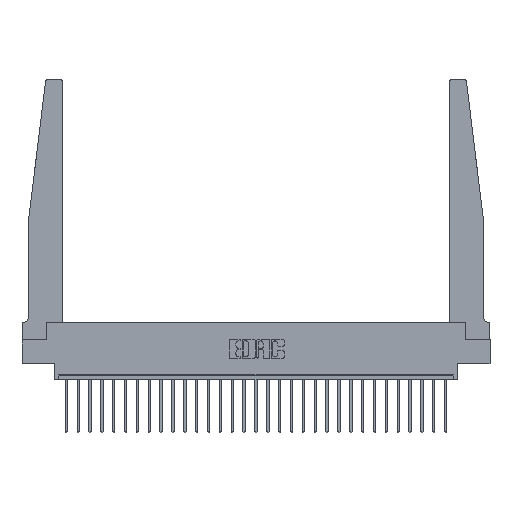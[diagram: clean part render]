
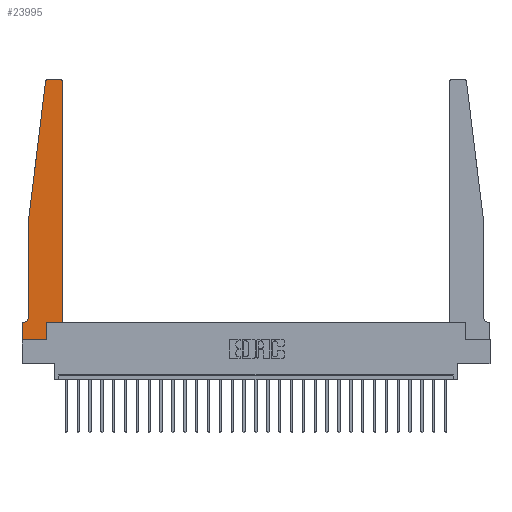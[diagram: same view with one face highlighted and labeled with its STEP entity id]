
A CAD part, top view. The second image highlights one B-rep face of the part: STEP entity #23995.
In plain terms, the highlighted planar face has unit normal (0, 0, 1).
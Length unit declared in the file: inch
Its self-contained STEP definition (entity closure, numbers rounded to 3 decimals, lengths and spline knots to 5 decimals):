
#101 = CARTESIAN_POINT ( 'NONE',  ( 0.015, 0.2375, 0.37 ) ) ;
#1660 = VECTOR ( 'NONE', #21999, 39.37008 ) ;
#1865 = LINE ( 'NONE', #8433, #6281 ) ;
#2936 = CARTESIAN_POINT ( 'NONE',  ( 0.065, 1.25, 0.37 ) ) ;
#2946 = LINE ( 'NONE', #7080, #1660 ) ;
#3023 = ORIENTED_EDGE ( 'NONE', *, *, #16589, .T. ) ;
#3166 = EDGE_CURVE ( 'NONE', #19661, #25735, #9652, .T. ) ;
#3373 = LINE ( 'NONE', #8254, #14221 ) ;
#3953 = EDGE_CURVE ( 'NONE', #21779, #18473, #4780, .T. ) ;
#4125 = CARTESIAN_POINT ( 'NONE',  ( 0., 0., 0.37 ) ) ;
#4203 = ORIENTED_EDGE ( 'NONE', *, *, #14254, .T. ) ;
#4204 = DIRECTION ( 'NONE',  ( -1., 0., 0. ) ) ;
#4245 = VECTOR ( 'NONE', #25683, 39.37008 ) ;
#4384 = VERTEX_POINT ( 'NONE', #24388 ) ;
#4780 = LINE ( 'NONE', #13141, #4907 ) ;
#4907 = VECTOR ( 'NONE', #21524, 39.37008 ) ;
#5101 = ORIENTED_EDGE ( 'NONE', *, *, #3953, .T. ) ;
#5239 = EDGE_CURVE ( 'NONE', #18473, #20666, #6199, .T. ) ;
#5373 = DIRECTION ( 'NONE',  ( 0., 0., 1. ) ) ;
#5426 = DIRECTION ( 'NONE',  ( 0., -1., 0. ) ) ;
#5432 = LINE ( 'NONE', #22148, #23500 ) ;
#5600 = VECTOR ( 'NONE', #7526, 39.37008 ) ;
#5661 = DIRECTION ( 'NONE',  ( 1., 0., 0. ) ) ;
#5679 = CARTESIAN_POINT ( 'NONE',  ( 0., 0., 0.37 ) ) ;
#6199 = LINE ( 'NONE', #4125, #15428 ) ;
#6280 = DIRECTION ( 'NONE',  ( 0., 0., -1. ) ) ;
#6281 = VECTOR ( 'NONE', #24971, 39.37008 ) ;
#6292 = DIRECTION ( 'NONE',  ( 1., 0., 0. ) ) ;
#7080 = CARTESIAN_POINT ( 'NONE',  ( 0.2605, 0.18, 0.37 ) ) ;
#7526 = DIRECTION ( 'NONE',  ( -1., 0., 0. ) ) ;
#7757 = VERTEX_POINT ( 'NONE', #9210 ) ;
#8254 = CARTESIAN_POINT ( 'NONE',  ( 0.065, 1.25, 0.37 ) ) ;
#8343 = CARTESIAN_POINT ( 'NONE',  ( 0.2605, 0.18, 0.37 ) ) ;
#8433 = CARTESIAN_POINT ( 'NONE',  ( 0.425, 0.18, 0.37 ) ) ;
#9161 = VECTOR ( 'NONE', #5661, 39.37008 ) ;
#9210 = CARTESIAN_POINT ( 'NONE',  ( 0.065, 0.2375, 0.37 ) ) ;
#9436 = AXIS2_PLACEMENT_3D ( 'NONE', #11283, #17607, #25920 ) ;
#9564 = LINE ( 'NONE', #26242, #5600 ) ;
#9652 = CIRCLE ( 'NONE', #13168, 0.03 ) ;
#10491 = CARTESIAN_POINT ( 'NONE',  ( 0.425, 2.72, 0.37 ) ) ;
#10650 = VERTEX_POINT ( 'NONE', #2936 ) ;
#10779 = DIRECTION ( 'NONE',  ( 0., 0., 1. ) ) ;
#10784 = EDGE_LOOP ( 'NONE', ( #18239, #18082, #24838, #4203, #22296, #5101, #16440, #13795, #3023, #15134, #13381, #20761 ) ) ;
#10858 = VERTEX_POINT ( 'NONE', #10491 ) ;
#10872 = EDGE_CURVE ( 'NONE', #7757, #21779, #24179, .T. ) ;
#10922 = PLANE ( 'NONE',  #18809 ) ;
#11168 = EDGE_CURVE ( 'NONE', #24058, #11967, #1865, .T. ) ;
#11248 = CARTESIAN_POINT ( 'NONE',  ( 0.27653, 2.75, 0.37 ) ) ;
#11283 = CARTESIAN_POINT ( 'NONE',  ( 0.395, 2.72, 0.37 ) ) ;
#11967 = VERTEX_POINT ( 'NONE', #13447 ) ;
#12859 = CARTESIAN_POINT ( 'NONE',  ( 0., 0.1875, 0.37 ) ) ;
#12895 = DIRECTION ( 'NONE',  ( 0., -1., 0. ) ) ;
#13141 = CARTESIAN_POINT ( 'NONE',  ( 0.065, 0.1875, 0.37 ) ) ;
#13168 = AXIS2_PLACEMENT_3D ( 'NONE', #20211, #5373, #19806 ) ;
#13298 = CARTESIAN_POINT ( 'NONE',  ( 0.395, 2.75, 0.37 ) ) ;
#13381 = ORIENTED_EDGE ( 'NONE', *, *, #21760, .T. ) ;
#13386 = LINE ( 'NONE', #19452, #4245 ) ;
#13447 = CARTESIAN_POINT ( 'NONE',  ( 0.425, 0.18, 0.37 ) ) ;
#13795 = ORIENTED_EDGE ( 'NONE', *, *, #13977, .T. ) ;
#13977 = EDGE_CURVE ( 'NONE', #20666, #4384, #16062, .T. ) ;
#14221 = VECTOR ( 'NONE', #5426, 39.37008 ) ;
#14254 = EDGE_CURVE ( 'NONE', #10650, #7757, #3373, .T. ) ;
#14568 = EDGE_CURVE ( 'NONE', #10858, #25699, #19537, .T. ) ;
#15134 = ORIENTED_EDGE ( 'NONE', *, *, #11168, .T. ) ;
#15428 = VECTOR ( 'NONE', #12895, 39.37008 ) ;
#15886 = AXIS2_PLACEMENT_3D ( 'NONE', #101, #6280, #4204 ) ;
#16062 = LINE ( 'NONE', #24386, #9161 ) ;
#16440 = ORIENTED_EDGE ( 'NONE', *, *, #5239, .T. ) ;
#16589 = EDGE_CURVE ( 'NONE', #4384, #24058, #2946, .T. ) ;
#17607 = DIRECTION ( 'NONE',  ( 0., 0., 1. ) ) ;
#18062 = DIRECTION ( 'NONE',  ( 0., 1., 0. ) ) ;
#18082 = ORIENTED_EDGE ( 'NONE', *, *, #3166, .T. ) ;
#18239 = ORIENTED_EDGE ( 'NONE', *, *, #22589, .T. ) ;
#18473 = VERTEX_POINT ( 'NONE', #27048 ) ;
#18809 = AXIS2_PLACEMENT_3D ( 'NONE', #12859, #10779, #6292 ) ;
#19452 = CARTESIAN_POINT ( 'NONE',  ( 0.065, 1.25, 0.37 ) ) ;
#19537 = CIRCLE ( 'NONE', #9436, 0.03 ) ;
#19661 = VERTEX_POINT ( 'NONE', #11248 ) ;
#19806 = DIRECTION ( 'NONE',  ( 1., 0., 0. ) ) ;
#20211 = CARTESIAN_POINT ( 'NONE',  ( 0.27653, 2.72, 0.37 ) ) ;
#20666 = VERTEX_POINT ( 'NONE', #5679 ) ;
#20761 = ORIENTED_EDGE ( 'NONE', *, *, #14568, .T. ) ;
#21524 = DIRECTION ( 'NONE',  ( -1., 0., 0. ) ) ;
#21607 = EDGE_CURVE ( 'NONE', #25735, #10650, #13386, .T. ) ;
#21760 = EDGE_CURVE ( 'NONE', #11967, #10858, #5432, .T. ) ;
#21779 = VERTEX_POINT ( 'NONE', #22276 ) ;
#21933 = CARTESIAN_POINT ( 'NONE',  ( 0.24675, 2.72367, 0.37 ) ) ;
#21999 = DIRECTION ( 'NONE',  ( 0., 1., 0. ) ) ;
#22148 = CARTESIAN_POINT ( 'NONE',  ( 0.425, 0.18, 0.37 ) ) ;
#22276 = CARTESIAN_POINT ( 'NONE',  ( 0.015, 0.1875, 0.37 ) ) ;
#22296 = ORIENTED_EDGE ( 'NONE', *, *, #10872, .T. ) ;
#22589 = EDGE_CURVE ( 'NONE', #25699, #19661, #9564, .T. ) ;
#23254 = FACE_OUTER_BOUND ( 'NONE', #10784, .T. ) ;
#23500 = VECTOR ( 'NONE', #18062, 39.37008 ) ;
#23995 = ADVANCED_FACE ( 'NONE', ( #23254 ), #10922, .T. ) ;
#24058 = VERTEX_POINT ( 'NONE', #8343 ) ;
#24179 = CIRCLE ( 'NONE', #15886, 0.05 ) ;
#24386 = CARTESIAN_POINT ( 'NONE',  ( 0., 0., 0.37 ) ) ;
#24388 = CARTESIAN_POINT ( 'NONE',  ( 0.2605, 0., 0.37 ) ) ;
#24838 = ORIENTED_EDGE ( 'NONE', *, *, #21607, .T. ) ;
#24971 = DIRECTION ( 'NONE',  ( 1., 0., 0. ) ) ;
#25683 = DIRECTION ( 'NONE',  ( -0.122, -0.992, 0. ) ) ;
#25699 = VERTEX_POINT ( 'NONE', #13298 ) ;
#25735 = VERTEX_POINT ( 'NONE', #21933 ) ;
#25920 = DIRECTION ( 'NONE',  ( 1., 0., 0. ) ) ;
#26242 = CARTESIAN_POINT ( 'NONE',  ( 0.25, 2.75, 0.37 ) ) ;
#27048 = CARTESIAN_POINT ( 'NONE',  ( 0., 0.1875, 0.37 ) ) ;
